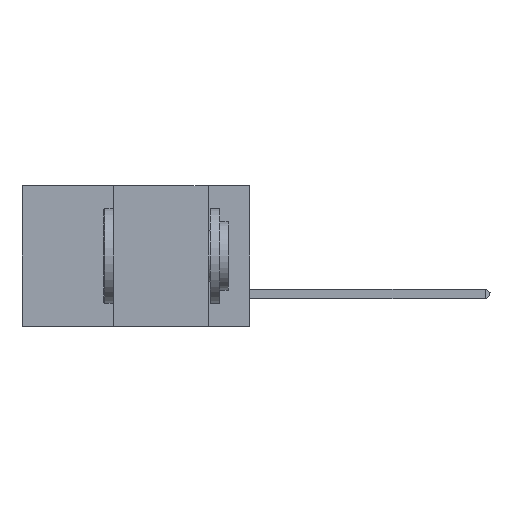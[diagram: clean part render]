
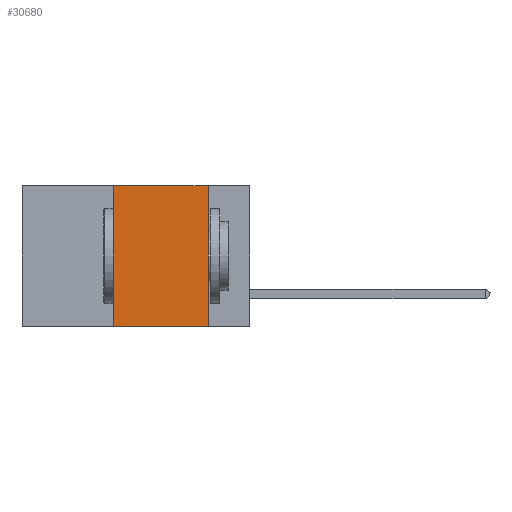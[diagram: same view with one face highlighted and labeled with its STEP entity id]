
A CAD part, left-side view. The second image highlights one B-rep face of the part: STEP entity #30680.
In plain terms, the highlighted planar face has unit normal (-1, 0, 0).
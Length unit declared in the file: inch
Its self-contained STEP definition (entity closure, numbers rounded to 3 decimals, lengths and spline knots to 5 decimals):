
#436 = VECTOR ( 'NONE', #45599, 39.37008 ) ;
#3186 = ORIENTED_EDGE ( 'NONE', *, *, #21187, .F. ) ;
#4483 = AXIS2_PLACEMENT_3D ( 'NONE', #46593, #17932, #28625 ) ;
#4977 = ORIENTED_EDGE ( 'NONE', *, *, #26308, .F. ) ;
#5676 = EDGE_CURVE ( 'NONE', #26927, #30581, #34853, .T. ) ;
#9685 = CARTESIAN_POINT ( 'NONE',  ( 0., 0.36, 0. ) ) ;
#11459 = CARTESIAN_POINT ( 'NONE',  ( 0., 0.11, -0.37 ) ) ;
#12720 = EDGE_LOOP ( 'NONE', ( #3186, #4977, #22048, #39065 ) ) ;
#14512 = VECTOR ( 'NONE', #38466, 39.37008 ) ;
#15862 = VERTEX_POINT ( 'NONE', #11459 ) ;
#17150 = CARTESIAN_POINT ( 'NONE',  ( 0., 0.36, -0.37 ) ) ;
#17788 = CARTESIAN_POINT ( 'NONE',  ( 0., 0.11, 0. ) ) ;
#17932 = DIRECTION ( 'NONE',  ( 1., 0., 0. ) ) ;
#18901 = DIRECTION ( 'NONE',  ( 0., -1., 0. ) ) ;
#20389 = CARTESIAN_POINT ( 'NONE',  ( 0., 0.11, 0. ) ) ;
#20886 = VECTOR ( 'NONE', #24828, 39.37008 ) ;
#21187 = EDGE_CURVE ( 'NONE', #30716, #15862, #39873, .T. ) ;
#21697 = PLANE ( 'NONE',  #4483 ) ;
#22048 = ORIENTED_EDGE ( 'NONE', *, *, #5676, .F. ) ;
#24828 = DIRECTION ( 'NONE',  ( 0., -1., 0. ) ) ;
#25281 = EDGE_CURVE ( 'NONE', #26927, #15862, #28726, .T. ) ;
#26308 = EDGE_CURVE ( 'NONE', #30581, #30716, #30446, .T. ) ;
#26927 = VERTEX_POINT ( 'NONE', #17150 ) ;
#27781 = CARTESIAN_POINT ( 'NONE',  ( 0., 0.36, 0. ) ) ;
#28625 = DIRECTION ( 'NONE',  ( 0., 0., -1. ) ) ;
#28726 = LINE ( 'NONE', #40353, #39466 ) ;
#30446 = LINE ( 'NONE', #32044, #20886 ) ;
#30581 = VERTEX_POINT ( 'NONE', #27781 ) ;
#30680 = ADVANCED_FACE ( 'NONE', ( #31154 ), #21697, .F. ) ;
#30716 = VERTEX_POINT ( 'NONE', #17788 ) ;
#31154 = FACE_OUTER_BOUND ( 'NONE', #12720, .T. ) ;
#32044 = CARTESIAN_POINT ( 'NONE',  ( 0., 0.6, 0. ) ) ;
#34853 = LINE ( 'NONE', #9685, #14512 ) ;
#38466 = DIRECTION ( 'NONE',  ( 0., 0., 1. ) ) ;
#39065 = ORIENTED_EDGE ( 'NONE', *, *, #25281, .T. ) ;
#39466 = VECTOR ( 'NONE', #18901, 39.37008 ) ;
#39873 = LINE ( 'NONE', #20389, #436 ) ;
#40353 = CARTESIAN_POINT ( 'NONE',  ( 0., 0.6, -0.37 ) ) ;
#45599 = DIRECTION ( 'NONE',  ( 0., 0., -1. ) ) ;
#46593 = CARTESIAN_POINT ( 'NONE',  ( 0., 0.6, 0. ) ) ;
